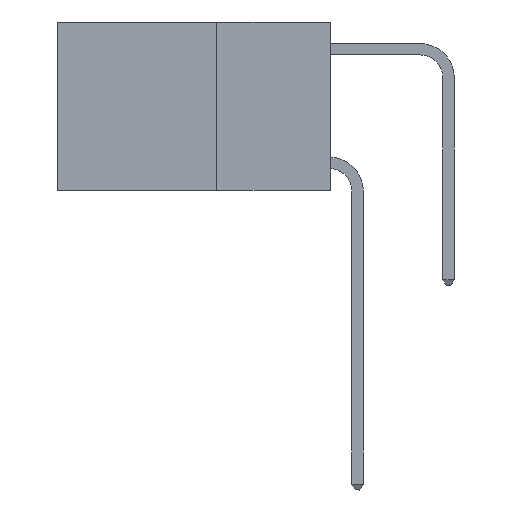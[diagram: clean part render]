
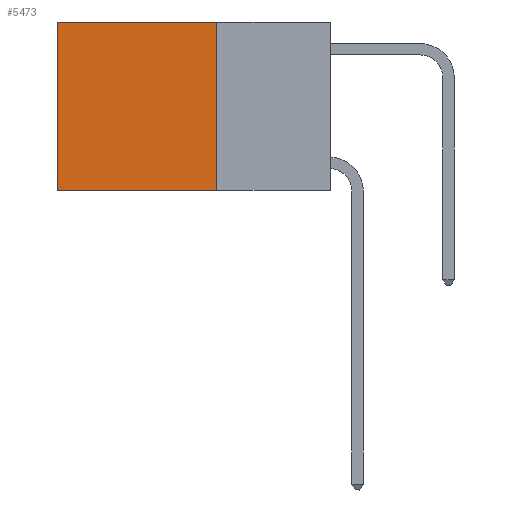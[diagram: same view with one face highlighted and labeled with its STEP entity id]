
A CAD part, left-side view. The second image highlights one B-rep face of the part: STEP entity #5473.
In plain terms, the highlighted planar face has unit normal (-1, 0, 0).
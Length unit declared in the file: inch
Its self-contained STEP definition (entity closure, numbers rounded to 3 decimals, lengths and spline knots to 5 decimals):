
#4549 = CARTESIAN_POINT ( 'NONE',  ( 0.2625, 0.25, -0.37 ) ) ;
#4553 = EDGE_CURVE ( 'NONE', #25297, #28914, #10458, .T. ) ;
#4710 = VERTEX_POINT ( 'NONE', #20719 ) ;
#4834 = DIRECTION ( 'NONE',  ( 1., 0., 0. ) ) ;
#5473 = ADVANCED_FACE ( 'NONE', ( #18958 ), #16941, .F. ) ;
#6685 = ORIENTED_EDGE ( 'NONE', *, *, #23395, .F. ) ;
#7149 = CARTESIAN_POINT ( 'NONE',  ( 0.2625, 0.25, 0. ) ) ;
#7621 = VECTOR ( 'NONE', #11651, 39.37008 ) ;
#8421 = AXIS2_PLACEMENT_3D ( 'NONE', #7149, #4834, #26429 ) ;
#9557 = EDGE_CURVE ( 'NONE', #16160, #4710, #24108, .T. ) ;
#10334 = CARTESIAN_POINT ( 'NONE',  ( 0.2625, 0.6, -0.37 ) ) ;
#10458 = LINE ( 'NONE', #20109, #29221 ) ;
#11651 = DIRECTION ( 'NONE',  ( 0., 0., -1. ) ) ;
#12515 = CARTESIAN_POINT ( 'NONE',  ( 0.2625, 0.25, 0. ) ) ;
#13757 = CARTESIAN_POINT ( 'NONE',  ( 0.2625, 0.25, 0. ) ) ;
#16160 = VERTEX_POINT ( 'NONE', #13757 ) ;
#16941 = PLANE ( 'NONE',  #8421 ) ;
#17134 = EDGE_LOOP ( 'NONE', ( #30668, #6685, #21555, #17799 ) ) ;
#17799 = ORIENTED_EDGE ( 'NONE', *, *, #28823, .T. ) ;
#18958 = FACE_OUTER_BOUND ( 'NONE', #17134, .T. ) ;
#20109 = CARTESIAN_POINT ( 'NONE',  ( 0.2625, 0.6, 0. ) ) ;
#20719 = CARTESIAN_POINT ( 'NONE',  ( 0.2625, 0.25, -0.37 ) ) ;
#21380 = VECTOR ( 'NONE', #28713, 39.37008 ) ;
#21555 = ORIENTED_EDGE ( 'NONE', *, *, #9557, .F. ) ;
#22172 = CARTESIAN_POINT ( 'NONE',  ( 0.2625, 0.6, 0. ) ) ;
#23395 = EDGE_CURVE ( 'NONE', #4710, #28914, #23788, .T. ) ;
#23788 = LINE ( 'NONE', #4549, #27222 ) ;
#24108 = LINE ( 'NONE', #25828, #7621 ) ;
#25297 = VERTEX_POINT ( 'NONE', #22172 ) ;
#25828 = CARTESIAN_POINT ( 'NONE',  ( 0.2625, 0.25, 0. ) ) ;
#26122 = DIRECTION ( 'NONE',  ( 0., 1., 0. ) ) ;
#26429 = DIRECTION ( 'NONE',  ( 0., 0., -1. ) ) ;
#27005 = LINE ( 'NONE', #12515, #21380 ) ;
#27222 = VECTOR ( 'NONE', #26122, 39.37008 ) ;
#27427 = DIRECTION ( 'NONE',  ( 0., 0., -1. ) ) ;
#28713 = DIRECTION ( 'NONE',  ( 0., 1., 0. ) ) ;
#28823 = EDGE_CURVE ( 'NONE', #16160, #25297, #27005, .T. ) ;
#28914 = VERTEX_POINT ( 'NONE', #10334 ) ;
#29221 = VECTOR ( 'NONE', #27427, 39.37008 ) ;
#30668 = ORIENTED_EDGE ( 'NONE', *, *, #4553, .T. ) ;
